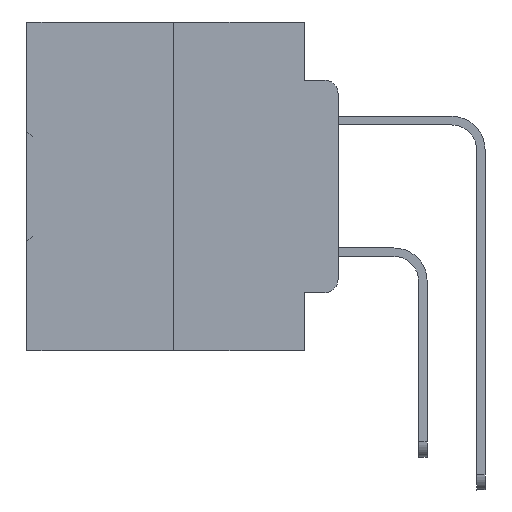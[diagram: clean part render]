
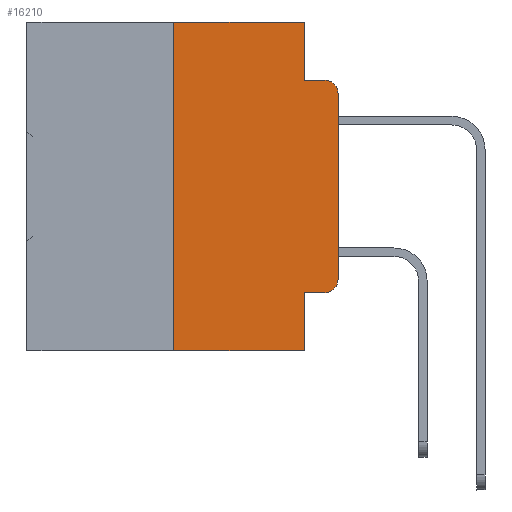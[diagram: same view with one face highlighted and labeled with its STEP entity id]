
A CAD part, left-side view. The second image highlights one B-rep face of the part: STEP entity #16210.
In plain terms, the highlighted planar face has unit normal (-1, 0, 0).
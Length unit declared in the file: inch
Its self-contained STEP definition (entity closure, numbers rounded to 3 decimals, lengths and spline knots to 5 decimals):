
#45 = VERTEX_POINT ( 'NONE', #249 ) ;
#226 = CIRCLE ( 'NONE', #33148, 0.02 ) ;
#249 = CARTESIAN_POINT ( 'NONE',  ( 0., 0.051, -0.0885 ) ) ;
#912 = VECTOR ( 'NONE', #14881, 39.37008 ) ;
#1170 = VERTEX_POINT ( 'NONE', #34629 ) ;
#1230 = CARTESIAN_POINT ( 'NONE',  ( 0., 0.473, 0. ) ) ;
#1375 = VECTOR ( 'NONE', #7847, 39.37008 ) ;
#1642 = CARTESIAN_POINT ( 'NONE',  ( 0., 0.473, 0. ) ) ;
#1672 = ORIENTED_EDGE ( 'NONE', *, *, #8118, .T. ) ;
#2249 = EDGE_CURVE ( 'NONE', #45, #11704, #21379, .T. ) ;
#2352 = VECTOR ( 'NONE', #34185, 39.37008 ) ;
#2677 = CARTESIAN_POINT ( 'NONE',  ( 0., 0., 0. ) ) ;
#2811 = LINE ( 'NONE', #29222, #912 ) ;
#3289 = CARTESIAN_POINT ( 'NONE',  ( 0., 0.02, -0.0885 ) ) ;
#4231 = DIRECTION ( 'NONE',  ( 0., 0., -1. ) ) ;
#4357 = CARTESIAN_POINT ( 'NONE',  ( 0., 0.02, -0.1085 ) ) ;
#4638 = DIRECTION ( 'NONE',  ( 0., -1., 0. ) ) ;
#5237 = LINE ( 'NONE', #23333, #12950 ) ;
#5943 = ORIENTED_EDGE ( 'NONE', *, *, #22311, .T. ) ;
#6117 = DIRECTION ( 'NONE',  ( 0., 0., -1. ) ) ;
#6180 = EDGE_CURVE ( 'NONE', #36452, #11704, #32650, .T. ) ;
#7246 = DIRECTION ( 'NONE',  ( 0., 0., -1. ) ) ;
#7679 = VECTOR ( 'NONE', #13692, 39.37008 ) ;
#7834 = VECTOR ( 'NONE', #4638, 39.37008 ) ;
#7847 = DIRECTION ( 'NONE',  ( 0., -1., 0. ) ) ;
#8118 = EDGE_CURVE ( 'NONE', #33301, #36452, #32939, .T. ) ;
#8225 = CARTESIAN_POINT ( 'NONE',  ( 0., 0.02, -0.3915 ) ) ;
#8613 = EDGE_CURVE ( 'NONE', #22222, #18706, #31151, .T. ) ;
#8773 = EDGE_LOOP ( 'NONE', ( #1672, #16950, #30048, #21041, #9476, #31255, #19677, #22367, #11121, #5943 ) ) ;
#9476 = ORIENTED_EDGE ( 'NONE', *, *, #31477, .F. ) ;
#11121 = ORIENTED_EDGE ( 'NONE', *, *, #24236, .T. ) ;
#11148 = DIRECTION ( 'NONE',  ( 0., 0., -1. ) ) ;
#11704 = VERTEX_POINT ( 'NONE', #3289 ) ;
#12427 = VECTOR ( 'NONE', #35698, 39.37008 ) ;
#12725 = PLANE ( 'NONE',  #30702 ) ;
#12950 = VECTOR ( 'NONE', #6117, 39.37008 ) ;
#13075 = CARTESIAN_POINT ( 'NONE',  ( 0., 0.051, -0.5 ) ) ;
#13094 = CARTESIAN_POINT ( 'NONE',  ( 0., 0.25, 0. ) ) ;
#13692 = DIRECTION ( 'NONE',  ( 0., -1., 0. ) ) ;
#14138 = VERTEX_POINT ( 'NONE', #20027 ) ;
#14881 = DIRECTION ( 'NONE',  ( 0., 0., 1. ) ) ;
#16013 = CARTESIAN_POINT ( 'NONE',  ( 0., 0.051, -0.0885 ) ) ;
#16210 = ADVANCED_FACE ( 'NONE', ( #33319 ), #12725, .F. ) ;
#16950 = ORIENTED_EDGE ( 'NONE', *, *, #6180, .T. ) ;
#18706 = VERTEX_POINT ( 'NONE', #13075 ) ;
#19677 = ORIENTED_EDGE ( 'NONE', *, *, #8613, .T. ) ;
#20027 = CARTESIAN_POINT ( 'NONE',  ( 0., 0.051, -0.4115 ) ) ;
#21041 = ORIENTED_EDGE ( 'NONE', *, *, #35682, .F. ) ;
#21113 = CARTESIAN_POINT ( 'NONE',  ( 0., 0., -0.3915 ) ) ;
#21379 = LINE ( 'NONE', #16013, #29003 ) ;
#21467 = DIRECTION ( 'NONE',  ( 1., 0., 0. ) ) ;
#22222 = VERTEX_POINT ( 'NONE', #33415 ) ;
#22311 = EDGE_CURVE ( 'NONE', #32654, #33301, #226, .T. ) ;
#22367 = ORIENTED_EDGE ( 'NONE', *, *, #28066, .F. ) ;
#22962 = LINE ( 'NONE', #33762, #7679 ) ;
#23333 = CARTESIAN_POINT ( 'NONE',  ( 0., 0.051, 0. ) ) ;
#24236 = EDGE_CURVE ( 'NONE', #14138, #32654, #22962, .T. ) ;
#24464 = DIRECTION ( 'NONE',  ( -1., 0., 0. ) ) ;
#26092 = CARTESIAN_POINT ( 'NONE',  ( 0., 0., -0.1085 ) ) ;
#26437 = VERTEX_POINT ( 'NONE', #13094 ) ;
#26895 = CARTESIAN_POINT ( 'NONE',  ( 0., 0.02, -0.4115 ) ) ;
#28066 = EDGE_CURVE ( 'NONE', #14138, #18706, #35196, .T. ) ;
#28299 = DIRECTION ( 'NONE',  ( -1., 0., 0. ) ) ;
#29003 = VECTOR ( 'NONE', #30251, 39.37008 ) ;
#29222 = CARTESIAN_POINT ( 'NONE',  ( 0., 0.25, 0. ) ) ;
#30048 = ORIENTED_EDGE ( 'NONE', *, *, #2249, .F. ) ;
#30251 = DIRECTION ( 'NONE',  ( 0., -1., 0. ) ) ;
#30694 = CARTESIAN_POINT ( 'NONE',  ( 0., 0.473, -0.5 ) ) ;
#30702 = AXIS2_PLACEMENT_3D ( 'NONE', #1230, #21467, #4231 ) ;
#30748 = LINE ( 'NONE', #1642, #7834 ) ;
#31151 = LINE ( 'NONE', #30694, #1375 ) ;
#31255 = ORIENTED_EDGE ( 'NONE', *, *, #31911, .F. ) ;
#31477 = EDGE_CURVE ( 'NONE', #26437, #1170, #30748, .T. ) ;
#31911 = EDGE_CURVE ( 'NONE', #22222, #26437, #2811, .T. ) ;
#32575 = AXIS2_PLACEMENT_3D ( 'NONE', #4357, #24464, #7246 ) ;
#32650 = CIRCLE ( 'NONE', #32575, 0.02 ) ;
#32654 = VERTEX_POINT ( 'NONE', #26895 ) ;
#32852 = CARTESIAN_POINT ( 'NONE',  ( 0., 0.051, 0. ) ) ;
#32939 = LINE ( 'NONE', #2677, #2352 ) ;
#33148 = AXIS2_PLACEMENT_3D ( 'NONE', #8225, #28299, #11148 ) ;
#33301 = VERTEX_POINT ( 'NONE', #21113 ) ;
#33319 = FACE_OUTER_BOUND ( 'NONE', #8773, .T. ) ;
#33415 = CARTESIAN_POINT ( 'NONE',  ( 0., 0.25, -0.5 ) ) ;
#33762 = CARTESIAN_POINT ( 'NONE',  ( 0., 0.051, -0.4115 ) ) ;
#34185 = DIRECTION ( 'NONE',  ( 0., 0., 1. ) ) ;
#34629 = CARTESIAN_POINT ( 'NONE',  ( 0., 0.051, 0. ) ) ;
#35196 = LINE ( 'NONE', #32852, #12427 ) ;
#35682 = EDGE_CURVE ( 'NONE', #1170, #45, #5237, .T. ) ;
#35698 = DIRECTION ( 'NONE',  ( 0., 0., -1. ) ) ;
#36452 = VERTEX_POINT ( 'NONE', #26092 ) ;
